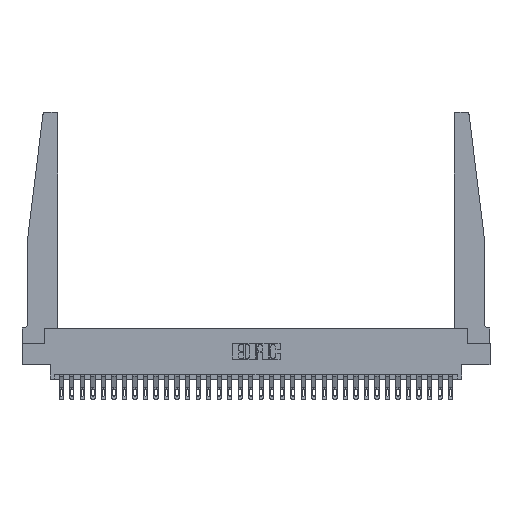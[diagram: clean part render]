
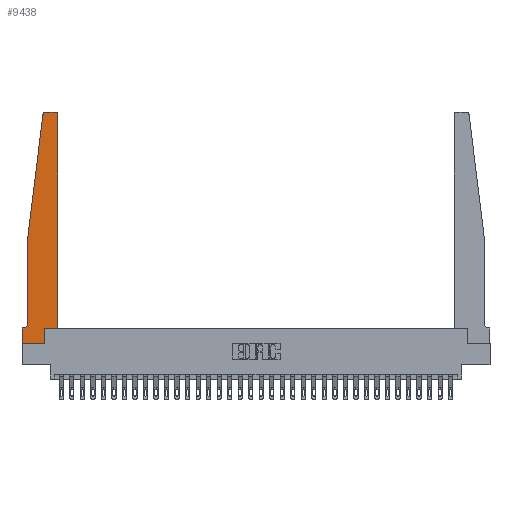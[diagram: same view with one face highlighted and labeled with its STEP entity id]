
A CAD part, top view. The second image highlights one B-rep face of the part: STEP entity #9438.
In plain terms, the highlighted planar face has unit normal (0, 0, 1).
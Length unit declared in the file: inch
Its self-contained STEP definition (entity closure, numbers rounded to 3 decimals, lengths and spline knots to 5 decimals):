
#61 = DIRECTION ( 'NONE',  ( 1., 0., 0. ) ) ;
#67 = VERTEX_POINT ( 'NONE', #19329 ) ;
#255 = CARTESIAN_POINT ( 'NONE',  ( 0.27653, 2.72, 0.37 ) ) ;
#272 = CARTESIAN_POINT ( 'NONE',  ( 0., 0.1875, 0.37 ) ) ;
#766 = VECTOR ( 'NONE', #14867, 39.37008 ) ;
#826 = ORIENTED_EDGE ( 'NONE', *, *, #29211, .T. ) ;
#976 = DIRECTION ( 'NONE',  ( 0., 0., -1. ) ) ;
#1252 = LINE ( 'NONE', #4967, #2011 ) ;
#1521 = LINE ( 'NONE', #21921, #766 ) ;
#2011 = VECTOR ( 'NONE', #19123, 39.37008 ) ;
#2397 = ORIENTED_EDGE ( 'NONE', *, *, #3948, .T. ) ;
#2654 = DIRECTION ( 'NONE',  ( 1., 0., 0. ) ) ;
#2847 = CARTESIAN_POINT ( 'NONE',  ( 0., 0., 0.37 ) ) ;
#3577 = VERTEX_POINT ( 'NONE', #18732 ) ;
#3674 = AXIS2_PLACEMENT_3D ( 'NONE', #272, #26316, #12268 ) ;
#3870 = ORIENTED_EDGE ( 'NONE', *, *, #20972, .T. ) ;
#3948 = EDGE_CURVE ( 'NONE', #67, #9568, #29500, .T. ) ;
#4319 = LINE ( 'NONE', #16331, #16193 ) ;
#4606 = CARTESIAN_POINT ( 'NONE',  ( 0.395, 2.72, 0.37 ) ) ;
#4644 = EDGE_CURVE ( 'NONE', #29147, #20155, #4774, .T. ) ;
#4709 = FACE_OUTER_BOUND ( 'NONE', #19080, .T. ) ;
#4774 = LINE ( 'NONE', #8062, #29834 ) ;
#4967 = CARTESIAN_POINT ( 'NONE',  ( 0.25, 2.75, 0.37 ) ) ;
#5716 = LINE ( 'NONE', #18422, #24512 ) ;
#5803 = CARTESIAN_POINT ( 'NONE',  ( 0.065, 1.25, 0.37 ) ) ;
#5839 = VERTEX_POINT ( 'NONE', #28655 ) ;
#6632 = ORIENTED_EDGE ( 'NONE', *, *, #7524, .T. ) ;
#6917 = DIRECTION ( 'NONE',  ( -0.122, -0.992, 0. ) ) ;
#6959 = LINE ( 'NONE', #19035, #30504 ) ;
#7008 = DIRECTION ( 'NONE',  ( 1., 0., 0. ) ) ;
#7524 = EDGE_CURVE ( 'NONE', #10664, #3577, #1252, .T. ) ;
#7530 = EDGE_CURVE ( 'NONE', #3577, #19223, #19424, .T. ) ;
#7690 = ORIENTED_EDGE ( 'NONE', *, *, #9356, .T. ) ;
#8062 = CARTESIAN_POINT ( 'NONE',  ( 0.425, 0.18, 0.37 ) ) ;
#8288 = ORIENTED_EDGE ( 'NONE', *, *, #7530, .T. ) ;
#9356 = EDGE_CURVE ( 'NONE', #5839, #10630, #6959, .T. ) ;
#9438 = ADVANCED_FACE ( 'NONE', ( #4709 ), #28575, .T. ) ;
#9568 = VERTEX_POINT ( 'NONE', #14946 ) ;
#10014 = AXIS2_PLACEMENT_3D ( 'NONE', #15220, #976, #17578 ) ;
#10579 = EDGE_CURVE ( 'NONE', #29262, #10664, #12811, .T. ) ;
#10630 = VERTEX_POINT ( 'NONE', #23576 ) ;
#10664 = VERTEX_POINT ( 'NONE', #23775 ) ;
#11130 = EDGE_CURVE ( 'NONE', #10630, #29147, #5716, .T. ) ;
#11457 = ORIENTED_EDGE ( 'NONE', *, *, #11130, .T. ) ;
#12268 = DIRECTION ( 'NONE',  ( 1., 0., 0. ) ) ;
#12811 = CIRCLE ( 'NONE', #29370, 0.03 ) ;
#12815 = DIRECTION ( 'NONE',  ( 1., 0., 0. ) ) ;
#14117 = EDGE_CURVE ( 'NONE', #18401, #5839, #20684, .T. ) ;
#14684 = VERTEX_POINT ( 'NONE', #21649 ) ;
#14867 = DIRECTION ( 'NONE',  ( 0., 1., 0. ) ) ;
#14946 = CARTESIAN_POINT ( 'NONE',  ( 0.015, 0.1875, 0.37 ) ) ;
#15220 = CARTESIAN_POINT ( 'NONE',  ( 0.015, 0.2375, 0.37 ) ) ;
#15267 = VECTOR ( 'NONE', #27038, 39.37008 ) ;
#15287 = ORIENTED_EDGE ( 'NONE', *, *, #10579, .T. ) ;
#15330 = VECTOR ( 'NONE', #19941, 39.37008 ) ;
#16193 = VECTOR ( 'NONE', #6917, 39.37008 ) ;
#16331 = CARTESIAN_POINT ( 'NONE',  ( 0.065, 1.25, 0.37 ) ) ;
#16875 = DIRECTION ( 'NONE',  ( 0., 0., 1. ) ) ;
#17070 = DIRECTION ( 'NONE',  ( 0., -1., 0. ) ) ;
#17396 = CARTESIAN_POINT ( 'NONE',  ( 0.2605, 0.18, 0.37 ) ) ;
#17578 = DIRECTION ( 'NONE',  ( -1., 0., 0. ) ) ;
#17872 = EDGE_CURVE ( 'NONE', #20155, #29262, #1521, .T. ) ;
#18003 = EDGE_CURVE ( 'NONE', #9568, #18401, #22238, .T. ) ;
#18401 = VERTEX_POINT ( 'NONE', #28557 ) ;
#18422 = CARTESIAN_POINT ( 'NONE',  ( 0.2605, 0.18, 0.37 ) ) ;
#18732 = CARTESIAN_POINT ( 'NONE',  ( 0.27653, 2.75, 0.37 ) ) ;
#18897 = ORIENTED_EDGE ( 'NONE', *, *, #17872, .T. ) ;
#19035 = CARTESIAN_POINT ( 'NONE',  ( 0., 0., 0.37 ) ) ;
#19080 = EDGE_LOOP ( 'NONE', ( #6632, #8288, #3870, #826, #2397, #19980, #25831, #7690, #11457, #21200, #18897, #15287 ) ) ;
#19123 = DIRECTION ( 'NONE',  ( -1., 0., 0. ) ) ;
#19223 = VERTEX_POINT ( 'NONE', #19493 ) ;
#19329 = CARTESIAN_POINT ( 'NONE',  ( 0.065, 0.2375, 0.37 ) ) ;
#19424 = CIRCLE ( 'NONE', #26201, 0.03 ) ;
#19493 = CARTESIAN_POINT ( 'NONE',  ( 0.24675, 2.72367, 0.37 ) ) ;
#19941 = DIRECTION ( 'NONE',  ( 0., -1., 0. ) ) ;
#19980 = ORIENTED_EDGE ( 'NONE', *, *, #18003, .T. ) ;
#20155 = VERTEX_POINT ( 'NONE', #22526 ) ;
#20684 = LINE ( 'NONE', #2847, #27658 ) ;
#20775 = DIRECTION ( 'NONE',  ( 0., 1., 0. ) ) ;
#20972 = EDGE_CURVE ( 'NONE', #19223, #14684, #4319, .T. ) ;
#21120 = DIRECTION ( 'NONE',  ( 0., 0., 1. ) ) ;
#21200 = ORIENTED_EDGE ( 'NONE', *, *, #4644, .T. ) ;
#21649 = CARTESIAN_POINT ( 'NONE',  ( 0.065, 1.25, 0.37 ) ) ;
#21921 = CARTESIAN_POINT ( 'NONE',  ( 0.425, 0.18, 0.37 ) ) ;
#22238 = LINE ( 'NONE', #24661, #15267 ) ;
#22526 = CARTESIAN_POINT ( 'NONE',  ( 0.425, 0.18, 0.37 ) ) ;
#23576 = CARTESIAN_POINT ( 'NONE',  ( 0.2605, 0., 0.37 ) ) ;
#23775 = CARTESIAN_POINT ( 'NONE',  ( 0.395, 2.75, 0.37 ) ) ;
#24512 = VECTOR ( 'NONE', #20775, 39.37008 ) ;
#24661 = CARTESIAN_POINT ( 'NONE',  ( 0.065, 0.1875, 0.37 ) ) ;
#25831 = ORIENTED_EDGE ( 'NONE', *, *, #14117, .T. ) ;
#26201 = AXIS2_PLACEMENT_3D ( 'NONE', #255, #16875, #2654 ) ;
#26316 = DIRECTION ( 'NONE',  ( 0., 0., 1. ) ) ;
#27038 = DIRECTION ( 'NONE',  ( -1., 0., 0. ) ) ;
#27658 = VECTOR ( 'NONE', #17070, 39.37008 ) ;
#27806 = LINE ( 'NONE', #5803, #15330 ) ;
#28557 = CARTESIAN_POINT ( 'NONE',  ( 0., 0.1875, 0.37 ) ) ;
#28575 = PLANE ( 'NONE',  #3674 ) ;
#28655 = CARTESIAN_POINT ( 'NONE',  ( 0., 0., 0.37 ) ) ;
#29147 = VERTEX_POINT ( 'NONE', #17396 ) ;
#29211 = EDGE_CURVE ( 'NONE', #14684, #67, #27806, .T. ) ;
#29262 = VERTEX_POINT ( 'NONE', #29472 ) ;
#29370 = AXIS2_PLACEMENT_3D ( 'NONE', #4606, #21120, #7008 ) ;
#29472 = CARTESIAN_POINT ( 'NONE',  ( 0.425, 2.72, 0.37 ) ) ;
#29500 = CIRCLE ( 'NONE', #10014, 0.05 ) ;
#29834 = VECTOR ( 'NONE', #12815, 39.37008 ) ;
#30504 = VECTOR ( 'NONE', #61, 39.37008 ) ;
